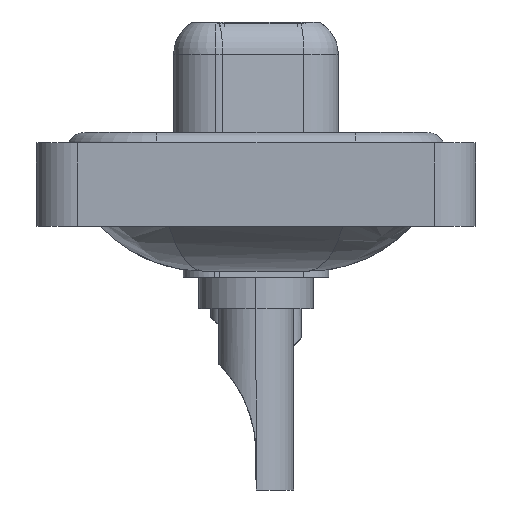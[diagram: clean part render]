
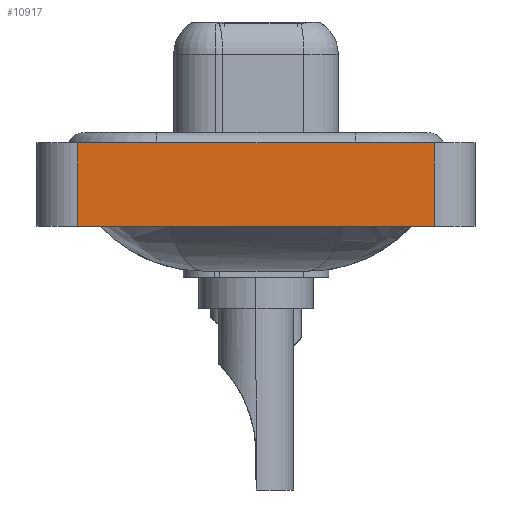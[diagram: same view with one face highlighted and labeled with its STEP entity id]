
A CAD part, left-side view. The second image highlights one B-rep face of the part: STEP entity #10917.
In plain terms, the highlighted planar face has unit normal (-1, 0, 0).
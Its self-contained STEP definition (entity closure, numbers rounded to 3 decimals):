
#836 = EDGE_LOOP ( 'NONE', ( #14349, #15180, #18936, #11830 ) ) ;
#1526 = VERTEX_POINT ( 'NONE', #2792 ) ;
#1959 = FACE_OUTER_BOUND ( 'NONE', #836, .T. ) ;
#1984 = CARTESIAN_POINT ( 'NONE',  ( -7.35, -8.55, 0.4 ) ) ;
#2036 = EDGE_CURVE ( 'NONE', #2211, #20136, #9237, .T. ) ;
#2211 = VERTEX_POINT ( 'NONE', #14459 ) ;
#2792 = CARTESIAN_POINT ( 'NONE',  ( -7.35, 8.55, -3.6 ) ) ;
#4866 = CARTESIAN_POINT ( 'NONE',  ( -7.35, -8.55, 0.4 ) ) ;
#5274 = DIRECTION ( 'NONE',  ( -1., 0., 0. ) ) ;
#6235 = VECTOR ( 'NONE', #20600, 1000. ) ;
#7400 = VECTOR ( 'NONE', #16933, 1000. ) ;
#7536 = EDGE_CURVE ( 'NONE', #20532, #20136, #12921, .T. ) ;
#8620 = CARTESIAN_POINT ( 'NONE',  ( -7.35, -8.55, -3.6 ) ) ;
#8646 = CARTESIAN_POINT ( 'NONE',  ( -7.35, -8.55, -3.6 ) ) ;
#9237 = LINE ( 'NONE', #18547, #7400 ) ;
#10047 = AXIS2_PLACEMENT_3D ( 'NONE', #8646, #5274, #19857 ) ;
#10427 = DIRECTION ( 'NONE',  ( 0., -1., 0. ) ) ;
#10917 = ADVANCED_FACE ( 'NONE', ( #1959 ), #13223, .T. ) ;
#10981 = CARTESIAN_POINT ( 'NONE',  ( -7.35, 8.55, -3.6 ) ) ;
#11224 = DIRECTION ( 'NONE',  ( 0., -1., 0. ) ) ;
#11830 = ORIENTED_EDGE ( 'NONE', *, *, #21045, .T. ) ;
#12921 = LINE ( 'NONE', #4866, #13431 ) ;
#13223 = PLANE ( 'NONE',  #10047 ) ;
#13327 = CARTESIAN_POINT ( 'NONE',  ( -7.35, 8.55, 0.4 ) ) ;
#13355 = EDGE_CURVE ( 'NONE', #1526, #20532, #20814, .T. ) ;
#13431 = VECTOR ( 'NONE', #11224, 1000. ) ;
#14349 = ORIENTED_EDGE ( 'NONE', *, *, #2036, .T. ) ;
#14459 = CARTESIAN_POINT ( 'NONE',  ( -7.35, -8.55, -3.6 ) ) ;
#15180 = ORIENTED_EDGE ( 'NONE', *, *, #7536, .F. ) ;
#15441 = LINE ( 'NONE', #8620, #17632 ) ;
#16933 = DIRECTION ( 'NONE',  ( 0., 0., 1. ) ) ;
#17632 = VECTOR ( 'NONE', #10427, 1000. ) ;
#18547 = CARTESIAN_POINT ( 'NONE',  ( -7.35, -8.55, -3.6 ) ) ;
#18936 = ORIENTED_EDGE ( 'NONE', *, *, #13355, .F. ) ;
#19857 = DIRECTION ( 'NONE',  ( 0., 0., 1. ) ) ;
#20136 = VERTEX_POINT ( 'NONE', #1984 ) ;
#20532 = VERTEX_POINT ( 'NONE', #13327 ) ;
#20600 = DIRECTION ( 'NONE',  ( 0., 0., 1. ) ) ;
#20814 = LINE ( 'NONE', #10981, #6235 ) ;
#21045 = EDGE_CURVE ( 'NONE', #1526, #2211, #15441, .T. ) ;
